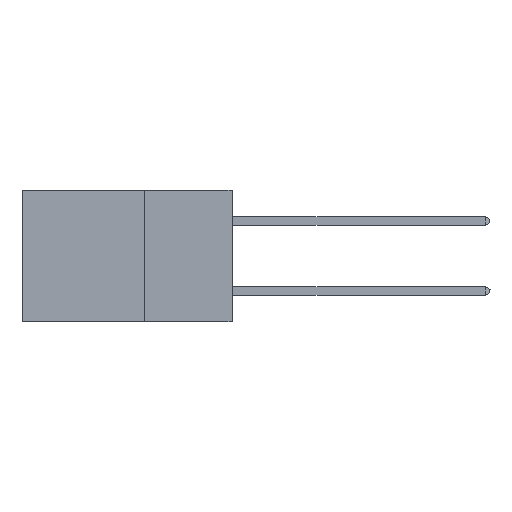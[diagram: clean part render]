
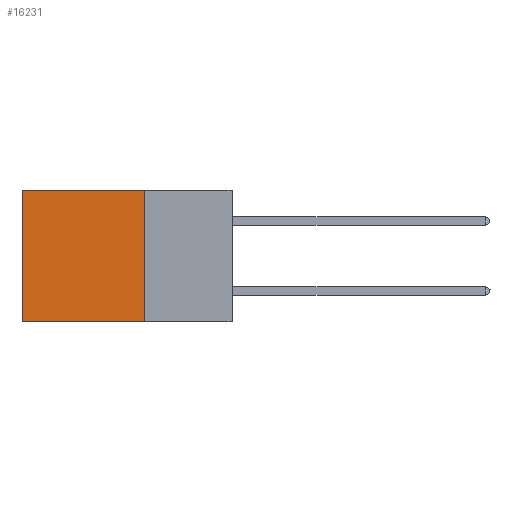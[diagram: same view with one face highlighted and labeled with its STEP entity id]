
A CAD part, left-side view. The second image highlights one B-rep face of the part: STEP entity #16231.
In plain terms, the highlighted planar face has unit normal (-1, 0, 0).
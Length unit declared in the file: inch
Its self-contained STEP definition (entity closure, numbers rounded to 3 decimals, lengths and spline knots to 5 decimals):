
#891 = ORIENTED_EDGE ( 'NONE', *, *, #9343, .T. ) ;
#1647 = EDGE_CURVE ( 'NONE', #9485, #8146, #8855, .T. ) ;
#1831 = LINE ( 'NONE', #20843, #13765 ) ;
#2433 = DIRECTION ( 'NONE',  ( 0., 1., 0. ) ) ;
#2695 = LINE ( 'NONE', #4046, #4278 ) ;
#3679 = CARTESIAN_POINT ( 'NONE',  ( 0.2875, 0.25, -0.375 ) ) ;
#4028 = CARTESIAN_POINT ( 'NONE',  ( 0.2875, 0.6, -0.375 ) ) ;
#4046 = CARTESIAN_POINT ( 'NONE',  ( 0.2875, 0.25, 0. ) ) ;
#4278 = VECTOR ( 'NONE', #2433, 39.37008 ) ;
#5142 = EDGE_CURVE ( 'NONE', #6776, #13575, #1831, .T. ) ;
#5748 = ORIENTED_EDGE ( 'NONE', *, *, #5142, .T. ) ;
#6776 = VERTEX_POINT ( 'NONE', #16639 ) ;
#8146 = VERTEX_POINT ( 'NONE', #3679 ) ;
#8158 = FACE_OUTER_BOUND ( 'NONE', #19707, .T. ) ;
#8783 = VECTOR ( 'NONE', #15980, 39.37008 ) ;
#8855 = LINE ( 'NONE', #11263, #13663 ) ;
#9343 = EDGE_CURVE ( 'NONE', #9485, #6776, #2695, .T. ) ;
#9485 = VERTEX_POINT ( 'NONE', #17527 ) ;
#10681 = PLANE ( 'NONE',  #19439 ) ;
#11263 = CARTESIAN_POINT ( 'NONE',  ( 0.2875, 0.25, -0.375 ) ) ;
#11661 = ORIENTED_EDGE ( 'NONE', *, *, #13911, .F. ) ;
#12393 = DIRECTION ( 'NONE',  ( 0., 0., -1. ) ) ;
#12607 = CARTESIAN_POINT ( 'NONE',  ( 0.2875, 0.25, -0.375 ) ) ;
#13575 = VERTEX_POINT ( 'NONE', #4028 ) ;
#13663 = VECTOR ( 'NONE', #17950, 39.37008 ) ;
#13765 = VECTOR ( 'NONE', #16221, 39.37008 ) ;
#13911 = EDGE_CURVE ( 'NONE', #8146, #13575, #16189, .T. ) ;
#14149 = CARTESIAN_POINT ( 'NONE',  ( 0.2875, 0.25, -0.375 ) ) ;
#14895 = ORIENTED_EDGE ( 'NONE', *, *, #1647, .F. ) ;
#15980 = DIRECTION ( 'NONE',  ( 0., 1., 0. ) ) ;
#16189 = LINE ( 'NONE', #14149, #8783 ) ;
#16221 = DIRECTION ( 'NONE',  ( 0., 0., -1. ) ) ;
#16231 = ADVANCED_FACE ( 'NONE', ( #8158 ), #10681, .F. ) ;
#16639 = CARTESIAN_POINT ( 'NONE',  ( 0.2875, 0.6, 0. ) ) ;
#17527 = CARTESIAN_POINT ( 'NONE',  ( 0.2875, 0.25, 0. ) ) ;
#17950 = DIRECTION ( 'NONE',  ( 0., 0., -1. ) ) ;
#19159 = DIRECTION ( 'NONE',  ( 1., 0., 0. ) ) ;
#19439 = AXIS2_PLACEMENT_3D ( 'NONE', #12607, #19159, #12393 ) ;
#19707 = EDGE_LOOP ( 'NONE', ( #5748, #11661, #14895, #891 ) ) ;
#20843 = CARTESIAN_POINT ( 'NONE',  ( 0.2875, 0.6, -0.375 ) ) ;
